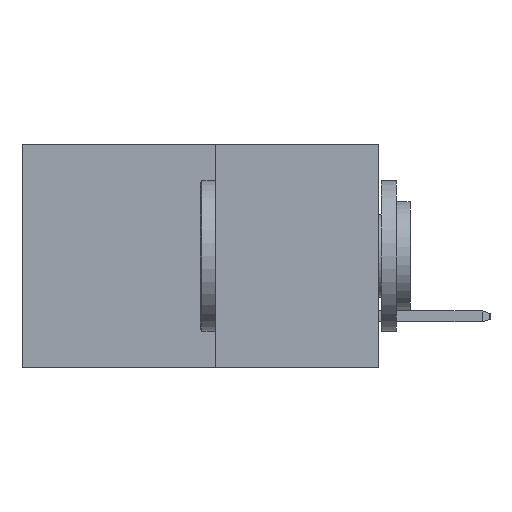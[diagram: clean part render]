
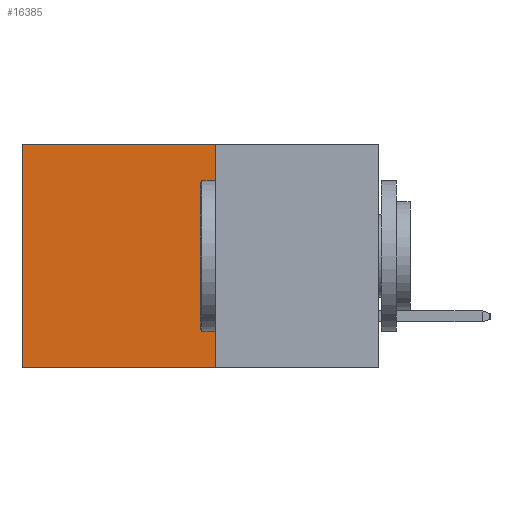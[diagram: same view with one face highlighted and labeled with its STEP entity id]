
A CAD part, left-side view. The second image highlights one B-rep face of the part: STEP entity #16385.
In plain terms, the highlighted planar face has unit normal (-1, 0, 0).
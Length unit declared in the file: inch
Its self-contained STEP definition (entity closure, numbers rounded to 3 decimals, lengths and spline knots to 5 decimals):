
#258 = DIRECTION ( 'NONE',  ( 0., 0., -1. ) ) ;
#587 = VERTEX_POINT ( 'NONE', #1333 ) ;
#1333 = CARTESIAN_POINT ( 'NONE',  ( 0.277, 0.59, 0. ) ) ;
#2353 = DIRECTION ( 'NONE',  ( 0., 1., 0. ) ) ;
#3143 = ORIENTED_EDGE ( 'NONE', *, *, #20674, .F. ) ;
#3576 = CARTESIAN_POINT ( 'NONE',  ( 0.277, 0.27, 0. ) ) ;
#3928 = DIRECTION ( 'NONE',  ( 0., 0., -1. ) ) ;
#4377 = CARTESIAN_POINT ( 'NONE',  ( 0.277, 0.27, -0.37 ) ) ;
#4704 = DIRECTION ( 'NONE',  ( 0., 0., -1. ) ) ;
#5249 = LINE ( 'NONE', #19730, #13445 ) ;
#5445 = VECTOR ( 'NONE', #2353, 39.37008 ) ;
#5569 = CARTESIAN_POINT ( 'NONE',  ( 0.277, 0.27, -0.37 ) ) ;
#5645 = VERTEX_POINT ( 'NONE', #4377 ) ;
#5927 = EDGE_LOOP ( 'NONE', ( #7402, #3143, #20829, #8879 ) ) ;
#6140 = EDGE_CURVE ( 'NONE', #15993, #5645, #7229, .T. ) ;
#7229 = LINE ( 'NONE', #5569, #19599 ) ;
#7402 = ORIENTED_EDGE ( 'NONE', *, *, #13920, .T. ) ;
#8879 = ORIENTED_EDGE ( 'NONE', *, *, #20089, .T. ) ;
#9891 = LINE ( 'NONE', #18553, #5445 ) ;
#11308 = CARTESIAN_POINT ( 'NONE',  ( 0.277, 0.27, -0.37 ) ) ;
#12902 = PLANE ( 'NONE',  #14305 ) ;
#13445 = VECTOR ( 'NONE', #258, 39.37008 ) ;
#13920 = EDGE_CURVE ( 'NONE', #587, #16325, #5249, .T. ) ;
#14305 = AXIS2_PLACEMENT_3D ( 'NONE', #11308, #14452, #4704 ) ;
#14452 = DIRECTION ( 'NONE',  ( 1., 0., 0. ) ) ;
#14965 = FACE_OUTER_BOUND ( 'NONE', #5927, .T. ) ;
#15375 = CARTESIAN_POINT ( 'NONE',  ( 0.277, 0.27, 0. ) ) ;
#15993 = VERTEX_POINT ( 'NONE', #3576 ) ;
#16325 = VERTEX_POINT ( 'NONE', #20650 ) ;
#16385 = ADVANCED_FACE ( 'NONE', ( #14965 ), #12902, .F. ) ;
#16979 = DIRECTION ( 'NONE',  ( 0., 1., 0. ) ) ;
#17652 = VECTOR ( 'NONE', #16979, 39.37008 ) ;
#18150 = LINE ( 'NONE', #15375, #17652 ) ;
#18553 = CARTESIAN_POINT ( 'NONE',  ( 0.277, 0.27, -0.37 ) ) ;
#19599 = VECTOR ( 'NONE', #3928, 39.37008 ) ;
#19730 = CARTESIAN_POINT ( 'NONE',  ( 0.277, 0.59, -0.37 ) ) ;
#20089 = EDGE_CURVE ( 'NONE', #15993, #587, #18150, .T. ) ;
#20650 = CARTESIAN_POINT ( 'NONE',  ( 0.277, 0.59, -0.37 ) ) ;
#20674 = EDGE_CURVE ( 'NONE', #5645, #16325, #9891, .T. ) ;
#20829 = ORIENTED_EDGE ( 'NONE', *, *, #6140, .F. ) ;
